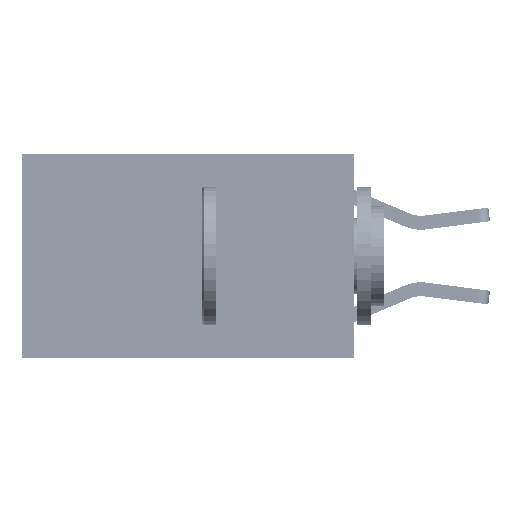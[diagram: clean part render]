
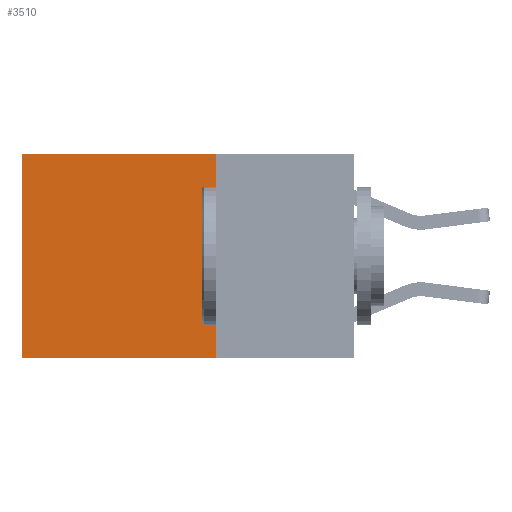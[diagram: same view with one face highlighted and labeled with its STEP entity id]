
A CAD part, left-side view. The second image highlights one B-rep face of the part: STEP entity #3510.
In plain terms, the highlighted planar face has unit normal (-1, 0, 0).
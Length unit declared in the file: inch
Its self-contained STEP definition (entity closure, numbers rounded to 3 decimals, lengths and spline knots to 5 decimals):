
#1331 = VECTOR ( 'NONE', #27494, 39.37008 ) ;
#1675 = CARTESIAN_POINT ( 'NONE',  ( 0.2625, 0.6, 0. ) ) ;
#2897 = LINE ( 'NONE', #7759, #1331 ) ;
#3510 = ADVANCED_FACE ( 'NONE', ( #31187 ), #18281, .F. ) ;
#3674 = VERTEX_POINT ( 'NONE', #21416 ) ;
#3971 = EDGE_CURVE ( 'NONE', #22927, #8727, #2897, .T. ) ;
#7759 = CARTESIAN_POINT ( 'NONE',  ( 0.2625, 0.25, -0.37 ) ) ;
#8482 = DIRECTION ( 'NONE',  ( 0., 0., -1. ) ) ;
#8705 = ORIENTED_EDGE ( 'NONE', *, *, #3971, .F. ) ;
#8727 = VERTEX_POINT ( 'NONE', #14023 ) ;
#9056 = CARTESIAN_POINT ( 'NONE',  ( 0.2625, 0.25, 0. ) ) ;
#9345 = DIRECTION ( 'NONE',  ( 0., 0., -1. ) ) ;
#9491 = VECTOR ( 'NONE', #14539, 39.37008 ) ;
#9523 = EDGE_CURVE ( 'NONE', #22454, #22927, #17684, .T. ) ;
#11375 = DIRECTION ( 'NONE',  ( 0., 1., 0. ) ) ;
#12327 = VECTOR ( 'NONE', #11375, 39.37008 ) ;
#14023 = CARTESIAN_POINT ( 'NONE',  ( 0.2625, 0.6, -0.37 ) ) ;
#14539 = DIRECTION ( 'NONE',  ( 0., 0., -1. ) ) ;
#14977 = LINE ( 'NONE', #1675, #28146 ) ;
#15037 = EDGE_LOOP ( 'NONE', ( #19021, #8705, #31765, #25660 ) ) ;
#15655 = DIRECTION ( 'NONE',  ( 1., 0., 0. ) ) ;
#17684 = LINE ( 'NONE', #29372, #9491 ) ;
#18281 = PLANE ( 'NONE',  #31235 ) ;
#18367 = CARTESIAN_POINT ( 'NONE',  ( 0.2625, 0.25, 0. ) ) ;
#19021 = ORIENTED_EDGE ( 'NONE', *, *, #21576, .T. ) ;
#20673 = EDGE_CURVE ( 'NONE', #22454, #3674, #23594, .T. ) ;
#21416 = CARTESIAN_POINT ( 'NONE',  ( 0.2625, 0.6, 0. ) ) ;
#21576 = EDGE_CURVE ( 'NONE', #3674, #8727, #14977, .T. ) ;
#22454 = VERTEX_POINT ( 'NONE', #9056 ) ;
#22927 = VERTEX_POINT ( 'NONE', #29340 ) ;
#23594 = LINE ( 'NONE', #23791, #12327 ) ;
#23791 = CARTESIAN_POINT ( 'NONE',  ( 0.2625, 0.25, 0. ) ) ;
#25660 = ORIENTED_EDGE ( 'NONE', *, *, #20673, .T. ) ;
#27494 = DIRECTION ( 'NONE',  ( 0., 1., 0. ) ) ;
#28146 = VECTOR ( 'NONE', #9345, 39.37008 ) ;
#29340 = CARTESIAN_POINT ( 'NONE',  ( 0.2625, 0.25, -0.37 ) ) ;
#29372 = CARTESIAN_POINT ( 'NONE',  ( 0.2625, 0.25, 0. ) ) ;
#31187 = FACE_OUTER_BOUND ( 'NONE', #15037, .T. ) ;
#31235 = AXIS2_PLACEMENT_3D ( 'NONE', #18367, #15655, #8482 ) ;
#31765 = ORIENTED_EDGE ( 'NONE', *, *, #9523, .F. ) ;
